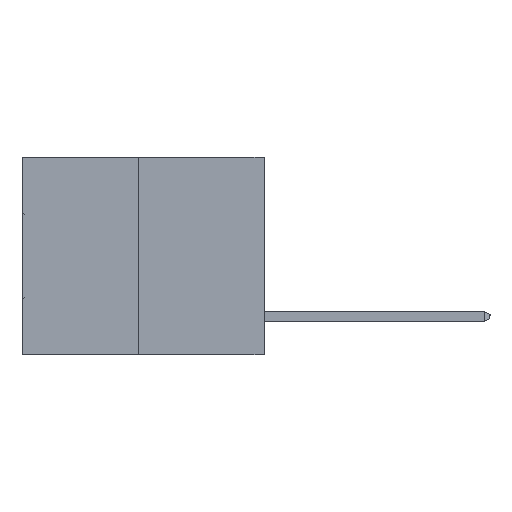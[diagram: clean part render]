
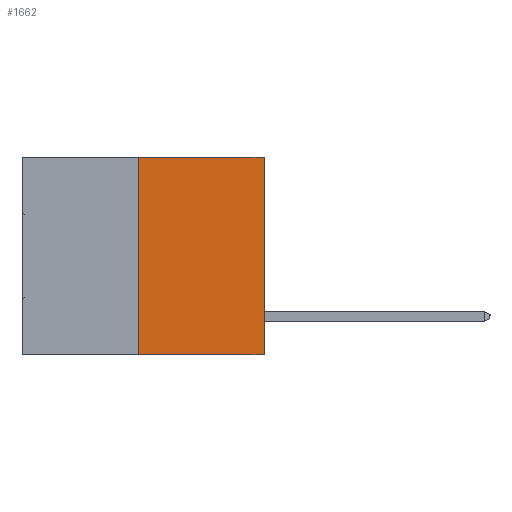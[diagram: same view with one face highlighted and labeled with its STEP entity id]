
A CAD part, left-side view. The second image highlights one B-rep face of the part: STEP entity #1662.
In plain terms, the highlighted planar face has unit normal (-1, 0, 0).
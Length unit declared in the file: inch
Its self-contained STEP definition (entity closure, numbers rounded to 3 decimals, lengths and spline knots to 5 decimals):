
#1175 = ORIENTED_EDGE ( 'NONE', *, *, #16006, .T. ) ;
#1662 = ADVANCED_FACE ( 'NONE', ( #31620 ), #23879, .F. ) ;
#1702 = CARTESIAN_POINT ( 'NONE',  ( 0., 0.6, -0.49 ) ) ;
#1893 = DIRECTION ( 'NONE',  ( 1., 0., 0. ) ) ;
#2737 = CARTESIAN_POINT ( 'NONE',  ( 0., 0.312, -0.49 ) ) ;
#4734 = DIRECTION ( 'NONE',  ( 0., 0., -1. ) ) ;
#7650 = ORIENTED_EDGE ( 'NONE', *, *, #32527, .T. ) ;
#7906 = VERTEX_POINT ( 'NONE', #15177 ) ;
#8270 = VECTOR ( 'NONE', #30683, 39.37008 ) ;
#8687 = VERTEX_POINT ( 'NONE', #23050 ) ;
#8936 = AXIS2_PLACEMENT_3D ( 'NONE', #21224, #1893, #4734 ) ;
#9576 = DIRECTION ( 'NONE',  ( 0., -1., 0. ) ) ;
#10336 = LINE ( 'NONE', #2737, #34723 ) ;
#11718 = ORIENTED_EDGE ( 'NONE', *, *, #28416, .F. ) ;
#12709 = CARTESIAN_POINT ( 'NONE',  ( 0., 0.312, 0. ) ) ;
#13684 = CARTESIAN_POINT ( 'NONE',  ( 0., 0., 0. ) ) ;
#14674 = VERTEX_POINT ( 'NONE', #33976 ) ;
#15177 = CARTESIAN_POINT ( 'NONE',  ( 0., 0., 0. ) ) ;
#15689 = LINE ( 'NONE', #13684, #8270 ) ;
#15985 = ORIENTED_EDGE ( 'NONE', *, *, #23578, .F. ) ;
#16006 = EDGE_CURVE ( 'NONE', #14674, #8687, #17151, .T. ) ;
#16624 = VERTEX_POINT ( 'NONE', #12709 ) ;
#17151 = LINE ( 'NONE', #1702, #35825 ) ;
#18603 = LINE ( 'NONE', #26100, #31628 ) ;
#21157 = DIRECTION ( 'NONE',  ( 0., -1., 0. ) ) ;
#21224 = CARTESIAN_POINT ( 'NONE',  ( 0., 0.6, 0. ) ) ;
#22043 = DIRECTION ( 'NONE',  ( 0., 0., 1. ) ) ;
#23050 = CARTESIAN_POINT ( 'NONE',  ( 0., 0., -0.49 ) ) ;
#23578 = EDGE_CURVE ( 'NONE', #14674, #16624, #10336, .T. ) ;
#23879 = PLANE ( 'NONE',  #8936 ) ;
#23929 = EDGE_LOOP ( 'NONE', ( #15985, #1175, #7650, #11718 ) ) ;
#26100 = CARTESIAN_POINT ( 'NONE',  ( 0., 0.6, 0. ) ) ;
#28416 = EDGE_CURVE ( 'NONE', #16624, #7906, #18603, .T. ) ;
#30683 = DIRECTION ( 'NONE',  ( 0., 0., 1. ) ) ;
#31620 = FACE_OUTER_BOUND ( 'NONE', #23929, .T. ) ;
#31628 = VECTOR ( 'NONE', #9576, 39.37008 ) ;
#32527 = EDGE_CURVE ( 'NONE', #8687, #7906, #15689, .T. ) ;
#33976 = CARTESIAN_POINT ( 'NONE',  ( 0., 0.312, -0.49 ) ) ;
#34723 = VECTOR ( 'NONE', #22043, 39.37008 ) ;
#35825 = VECTOR ( 'NONE', #21157, 39.37008 ) ;
